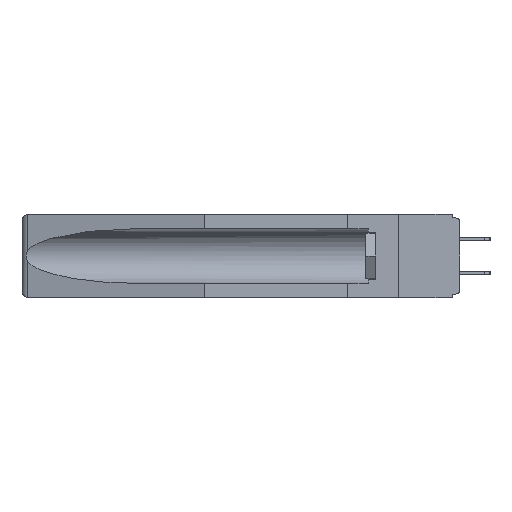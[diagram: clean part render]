
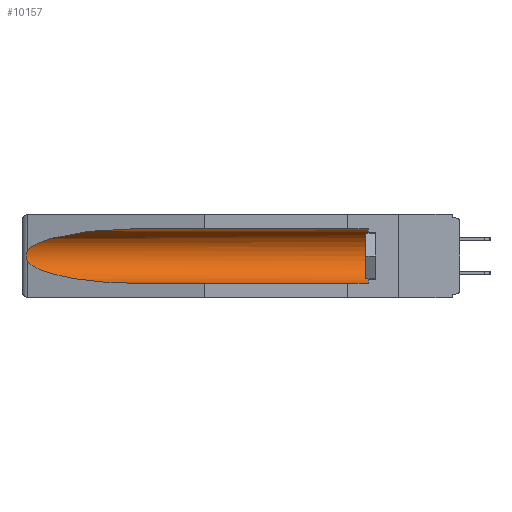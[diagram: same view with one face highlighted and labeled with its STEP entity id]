
A CAD part, left-side view. The second image highlights one B-rep face of the part: STEP entity #10157.
In plain terms, the highlighted cylindrical face has radius 2.857 mm (diameter 5.715 mm), a partial arc.
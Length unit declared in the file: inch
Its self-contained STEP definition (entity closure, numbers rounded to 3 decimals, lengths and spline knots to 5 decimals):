
#152 = CARTESIAN_POINT ( 'NONE',  ( 0.26537, 1.52718, -0.14972 ) ) ;
#645 = CARTESIAN_POINT ( 'NONE',  ( 0.2675, 1.53308, -0.17534 ) ) ;
#863 = CARTESIAN_POINT ( 'NONE',  ( 0.26597, 1.5296, -0.19026 ) ) ;
#900 = CARTESIAN_POINT ( 'NONE',  ( 0.26537, 1.52718, -0.14972 ) ) ;
#983 = CARTESIAN_POINT ( 'NONE',  ( 0.26655, 1.53094, -0.18657 ) ) ;
#2773 =( BOUNDED_CURVE ( )  B_SPLINE_CURVE ( 3, ( #25287, #27872, #23240, #23469 ),
 .UNSPECIFIED., .F., .F. ) 
 B_SPLINE_CURVE_WITH_KNOTS ( ( 4, 4 ),
 ( 0.1948, 1.5708 ),
 .UNSPECIFIED. ) 
 CURVE ( )  GEOMETRIC_REPRESENTATION_ITEM ( )  RATIONAL_B_SPLINE_CURVE ( ( 1., 0.848, 0.848, 1. ) ) 
 REPRESENTATION_ITEM ( '' )  );
#3384 = CARTESIAN_POINT ( 'NONE',  ( 0.26537, 1.52718, -0.19328 ) ) ;
#3957 = CARTESIAN_POINT ( 'NONE',  ( 0.155, 0.126, -0.059 ) ) ;
#6015 = CARTESIAN_POINT ( 'NONE',  ( 0.155, 0.126, -0.1715 ) ) ;
#6493 = EDGE_CURVE ( 'NONE', #11317, #17726, #13298, .T. ) ;
#7510 = VECTOR ( 'NONE', #23915, 39.37008 ) ;
#7538 = ORIENTED_EDGE ( 'NONE', *, *, #30703, .F. ) ;
#8216 = CARTESIAN_POINT ( 'NONE',  ( 0.21114, 1.30732, -0.059 ) ) ;
#8508 = DIRECTION ( 'NONE',  ( 0., -1., 0. ) ) ;
#8511 = CARTESIAN_POINT ( 'NONE',  ( 0.2673, 1.5327, -0.16383 ) ) ;
#9468 = ORIENTED_EDGE ( 'NONE', *, *, #25399, .T. ) ;
#10112 = VERTEX_POINT ( 'NONE', #26560 ) ;
#10157 = ADVANCED_FACE ( 'NONE', ( #16924 ), #16553, .F. ) ;
#10647 = ORIENTED_EDGE ( 'NONE', *, *, #11710, .T. ) ;
#11055 = CARTESIAN_POINT ( 'NONE',  ( 0.155, -0.30754, -0.059 ) ) ;
#11270 = CARTESIAN_POINT ( 'NONE',  ( 0.25451, 1.48313, -0.09465 ) ) ;
#11317 = VERTEX_POINT ( 'NONE', #13875 ) ;
#11710 = EDGE_CURVE ( 'NONE', #19456, #20620, #14199, .T. ) ;
#12299 = EDGE_CURVE ( 'NONE', #17726, #10112, #29294, .T. ) ;
#12410 = LINE ( 'NONE', #21321, #7510 ) ;
#13046 = ORIENTED_EDGE ( 'NONE', *, *, #12299, .T. ) ;
#13298 = CIRCLE ( 'NONE', #13680, 0.1125 ) ;
#13680 = AXIS2_PLACEMENT_3D ( 'NONE', #6015, #8508, #31817 ) ;
#13846 = CARTESIAN_POINT ( 'NONE',  ( 0.26537, 1.52718, -0.19328 ) ) ;
#13875 = CARTESIAN_POINT ( 'NONE',  ( 0.155, 0.126, -0.284 ) ) ;
#14199 = B_SPLINE_CURVE_WITH_KNOTS ( 'NONE', 3,
 ( #29261, #26453, #19025, #8511, #16121, #645, #29038, #983, #863, #13846 ),
 .UNSPECIFIED., .F., .F.,
 ( 4, 2, 2, 2, 4 ),
 ( 0., 0.00029, 0.00058, 0.00087, 0.00117 ),
 .UNSPECIFIED. ) ;
#14793 =( BOUNDED_CURVE ( )  B_SPLINE_CURVE ( 3, ( #16265, #8216, #11270, #900 ),
 .UNSPECIFIED., .F., .F. ) 
 B_SPLINE_CURVE_WITH_KNOTS ( ( 4, 4 ),
 ( 4.71239, 6.08839 ),
 .UNSPECIFIED. ) 
 CURVE ( )  GEOMETRIC_REPRESENTATION_ITEM ( )  RATIONAL_B_SPLINE_CURVE ( ( 1., 0.848, 0.848, 1. ) ) 
 REPRESENTATION_ITEM ( '' )  );
#16044 = EDGE_LOOP ( 'NONE', ( #22649, #10647, #9468, #7538, #27558, #13046 ) ) ;
#16121 = CARTESIAN_POINT ( 'NONE',  ( 0.2675, 1.53308, -0.16763 ) ) ;
#16265 = CARTESIAN_POINT ( 'NONE',  ( 0.155, 1.07973, -0.059 ) ) ;
#16553 = CYLINDRICAL_SURFACE ( 'NONE', #24565, 0.1125 ) ;
#16924 = FACE_OUTER_BOUND ( 'NONE', #16044, .T. ) ;
#17726 = VERTEX_POINT ( 'NONE', #3957 ) ;
#18947 = DIRECTION ( 'NONE',  ( 0., 0., 1. ) ) ;
#19025 = CARTESIAN_POINT ( 'NONE',  ( 0.26654, 1.53092, -0.15636 ) ) ;
#19456 = VERTEX_POINT ( 'NONE', #152 ) ;
#20620 = VERTEX_POINT ( 'NONE', #3384 ) ;
#21006 = DIRECTION ( 'NONE',  ( 0., 1., 0. ) ) ;
#21321 = CARTESIAN_POINT ( 'NONE',  ( 0.155, -0.30754, -0.284 ) ) ;
#22649 = ORIENTED_EDGE ( 'NONE', *, *, #25561, .T. ) ;
#23240 = CARTESIAN_POINT ( 'NONE',  ( 0.21114, 1.30732, -0.284 ) ) ;
#23469 = CARTESIAN_POINT ( 'NONE',  ( 0.155, 1.07973, -0.284 ) ) ;
#23915 = DIRECTION ( 'NONE',  ( 0., 1., 0. ) ) ;
#24070 = VERTEX_POINT ( 'NONE', #31230 ) ;
#24565 = AXIS2_PLACEMENT_3D ( 'NONE', #25866, #24737, #18947 ) ;
#24737 = DIRECTION ( 'NONE',  ( 0., 1., 0. ) ) ;
#24890 = VECTOR ( 'NONE', #21006, 39.37008 ) ;
#25287 = CARTESIAN_POINT ( 'NONE',  ( 0.26537, 1.52718, -0.19328 ) ) ;
#25399 = EDGE_CURVE ( 'NONE', #20620, #24070, #2773, .T. ) ;
#25561 = EDGE_CURVE ( 'NONE', #10112, #19456, #14793, .T. ) ;
#25866 = CARTESIAN_POINT ( 'NONE',  ( 0.155, -0.30754, -0.1715 ) ) ;
#26453 = CARTESIAN_POINT ( 'NONE',  ( 0.26597, 1.52961, -0.15275 ) ) ;
#26560 = CARTESIAN_POINT ( 'NONE',  ( 0.155, 1.07973, -0.059 ) ) ;
#27558 = ORIENTED_EDGE ( 'NONE', *, *, #6493, .T. ) ;
#27872 = CARTESIAN_POINT ( 'NONE',  ( 0.25451, 1.48313, -0.24835 ) ) ;
#29038 = CARTESIAN_POINT ( 'NONE',  ( 0.2673, 1.53269, -0.17917 ) ) ;
#29261 = CARTESIAN_POINT ( 'NONE',  ( 0.26537, 1.52718, -0.14972 ) ) ;
#29294 = LINE ( 'NONE', #11055, #24890 ) ;
#30703 = EDGE_CURVE ( 'NONE', #11317, #24070, #12410, .T. ) ;
#31230 = CARTESIAN_POINT ( 'NONE',  ( 0.155, 1.07973, -0.284 ) ) ;
#31817 = DIRECTION ( 'NONE',  ( 0., 0., 1. ) ) ;
